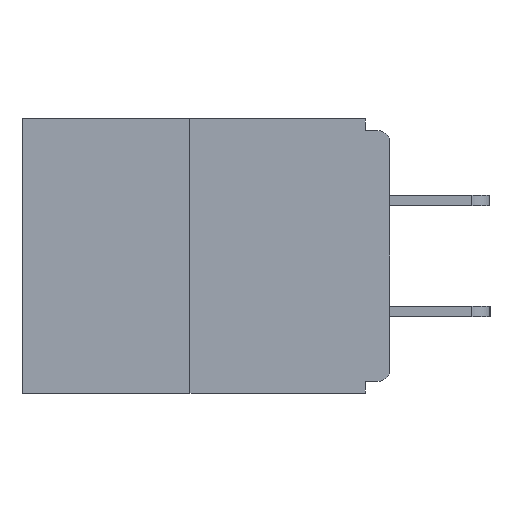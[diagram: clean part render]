
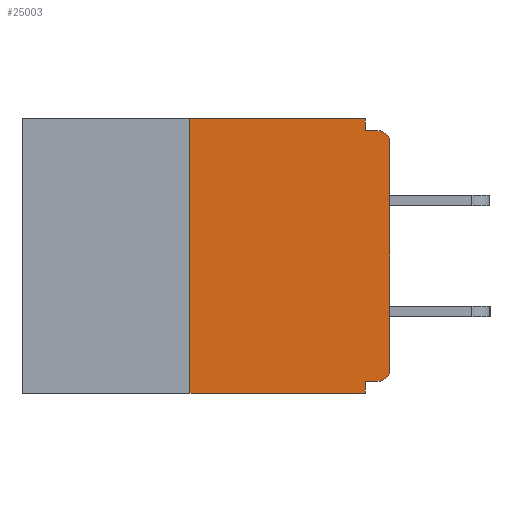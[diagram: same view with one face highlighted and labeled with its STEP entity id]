
A CAD part, left-side view. The second image highlights one B-rep face of the part: STEP entity #25003.
In plain terms, the highlighted planar face has unit normal (-1, 0, 0).
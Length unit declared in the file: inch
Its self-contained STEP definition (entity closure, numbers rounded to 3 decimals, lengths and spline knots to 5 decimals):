
#54 = VERTEX_POINT ( 'NONE', #17218 ) ;
#560 = VERTEX_POINT ( 'NONE', #18447 ) ;
#632 = CARTESIAN_POINT ( 'NONE',  ( 0., 0.25, -0.343 ) ) ;
#1004 = DIRECTION ( 'NONE',  ( 1., 0., 0. ) ) ;
#1020 = EDGE_CURVE ( 'NONE', #22884, #10326, #26032, .T. ) ;
#1209 = CARTESIAN_POINT ( 'NONE',  ( 0., 0.46, 0. ) ) ;
#1566 = ORIENTED_EDGE ( 'NONE', *, *, #19395, .F. ) ;
#1729 = CARTESIAN_POINT ( 'NONE',  ( 0., 0.015, -0.313 ) ) ;
#1945 = ORIENTED_EDGE ( 'NONE', *, *, #5148, .T. ) ;
#2674 = CARTESIAN_POINT ( 'NONE',  ( 0., 0., -0.328 ) ) ;
#2755 = DIRECTION ( 'NONE',  ( 0., 0., -1. ) ) ;
#2906 = LINE ( 'NONE', #23222, #14003 ) ;
#2956 = AXIS2_PLACEMENT_3D ( 'NONE', #24264, #5818, #22269 ) ;
#3060 = ORIENTED_EDGE ( 'NONE', *, *, #17266, .T. ) ;
#3271 = AXIS2_PLACEMENT_3D ( 'NONE', #5281, #1004, #7443 ) ;
#3299 = CARTESIAN_POINT ( 'NONE',  ( 0., 0., 0. ) ) ;
#3790 = VERTEX_POINT ( 'NONE', #10400 ) ;
#4500 = EDGE_CURVE ( 'NONE', #54, #8327, #11698, .T. ) ;
#4554 = VECTOR ( 'NONE', #18564, 39.37008 ) ;
#5148 = EDGE_CURVE ( 'NONE', #22478, #26376, #26455, .T. ) ;
#5281 = CARTESIAN_POINT ( 'NONE',  ( 0., 0.46, 0. ) ) ;
#5818 = DIRECTION ( 'NONE',  ( -1., 0., 0. ) ) ;
#7095 = VECTOR ( 'NONE', #7277, 39.37008 ) ;
#7277 = DIRECTION ( 'NONE',  ( 0., 0., -1. ) ) ;
#7323 = LINE ( 'NONE', #3299, #12209 ) ;
#7443 = DIRECTION ( 'NONE',  ( 0., 0., -1. ) ) ;
#7733 = EDGE_CURVE ( 'NONE', #8327, #25374, #17316, .T. ) ;
#7776 = CARTESIAN_POINT ( 'NONE',  ( 0., 0.46, -0.343 ) ) ;
#8327 = VERTEX_POINT ( 'NONE', #23055 ) ;
#8697 = EDGE_CURVE ( 'NONE', #22884, #560, #16909, .T. ) ;
#8846 = DIRECTION ( 'NONE',  ( 0., 1., 0. ) ) ;
#9107 = CARTESIAN_POINT ( 'NONE',  ( 0., 0., -0.015 ) ) ;
#9693 = ORIENTED_EDGE ( 'NONE', *, *, #1020, .T. ) ;
#10137 = VECTOR ( 'NONE', #20586, 39.37008 ) ;
#10212 = VECTOR ( 'NONE', #10858, 39.37008 ) ;
#10326 = VERTEX_POINT ( 'NONE', #21945 ) ;
#10337 = CARTESIAN_POINT ( 'NONE',  ( 0., 0.25, 0. ) ) ;
#10400 = CARTESIAN_POINT ( 'NONE',  ( 0., 0.25, 0. ) ) ;
#10466 = EDGE_CURVE ( 'NONE', #10326, #24249, #7323, .T. ) ;
#10858 = DIRECTION ( 'NONE',  ( 0., -1., 0. ) ) ;
#11034 = CARTESIAN_POINT ( 'NONE',  ( 0., 0., -0.03 ) ) ;
#11698 = LINE ( 'NONE', #23699, #7095 ) ;
#12086 = LINE ( 'NONE', #10337, #4554 ) ;
#12209 = VECTOR ( 'NONE', #12879, 39.37008 ) ;
#12280 = AXIS2_PLACEMENT_3D ( 'NONE', #1729, #13937, #18138 ) ;
#12622 = ORIENTED_EDGE ( 'NONE', *, *, #7733, .F. ) ;
#12879 = DIRECTION ( 'NONE',  ( 0., 0., 1. ) ) ;
#13374 = FACE_OUTER_BOUND ( 'NONE', #15676, .T. ) ;
#13558 = LINE ( 'NONE', #1209, #25602 ) ;
#13937 = DIRECTION ( 'NONE',  ( -1., 0., 0. ) ) ;
#14003 = VECTOR ( 'NONE', #2755, 39.37008 ) ;
#14537 = ORIENTED_EDGE ( 'NONE', *, *, #8697, .F. ) ;
#14550 = CIRCLE ( 'NONE', #2956, 0.015 ) ;
#15676 = EDGE_LOOP ( 'NONE', ( #16479, #1566, #1945, #21138, #14537, #9693, #23672, #3060, #12622, #23519 ) ) ;
#16479 = ORIENTED_EDGE ( 'NONE', *, *, #19364, .F. ) ;
#16909 = LINE ( 'NONE', #2674, #21766 ) ;
#17218 = CARTESIAN_POINT ( 'NONE',  ( 0., 0.031, 0. ) ) ;
#17266 = EDGE_CURVE ( 'NONE', #24249, #25374, #14550, .T. ) ;
#17316 = LINE ( 'NONE', #9107, #10212 ) ;
#17621 = DIRECTION ( 'NONE',  ( 0., -1., 0. ) ) ;
#17877 = CARTESIAN_POINT ( 'NONE',  ( 0., 0.015, -0.015 ) ) ;
#18138 = DIRECTION ( 'NONE',  ( 0., 0., -1. ) ) ;
#18189 = CARTESIAN_POINT ( 'NONE',  ( 0., 0.015, -0.328 ) ) ;
#18447 = CARTESIAN_POINT ( 'NONE',  ( 0., 0.031, -0.328 ) ) ;
#18564 = DIRECTION ( 'NONE',  ( 0., 0., 1. ) ) ;
#19364 = EDGE_CURVE ( 'NONE', #3790, #54, #13558, .T. ) ;
#19395 = EDGE_CURVE ( 'NONE', #22478, #3790, #12086, .T. ) ;
#19454 = PLANE ( 'NONE',  #3271 ) ;
#20586 = DIRECTION ( 'NONE',  ( 0., -1., 0. ) ) ;
#21138 = ORIENTED_EDGE ( 'NONE', *, *, #26142, .F. ) ;
#21766 = VECTOR ( 'NONE', #8846, 39.37008 ) ;
#21945 = CARTESIAN_POINT ( 'NONE',  ( 0., 0., -0.313 ) ) ;
#22269 = DIRECTION ( 'NONE',  ( 0., 0., -1. ) ) ;
#22478 = VERTEX_POINT ( 'NONE', #632 ) ;
#22884 = VERTEX_POINT ( 'NONE', #18189 ) ;
#23055 = CARTESIAN_POINT ( 'NONE',  ( 0., 0.031, -0.015 ) ) ;
#23222 = CARTESIAN_POINT ( 'NONE',  ( 0., 0.031, -0.343 ) ) ;
#23519 = ORIENTED_EDGE ( 'NONE', *, *, #4500, .F. ) ;
#23672 = ORIENTED_EDGE ( 'NONE', *, *, #10466, .T. ) ;
#23699 = CARTESIAN_POINT ( 'NONE',  ( 0., 0.031, 0. ) ) ;
#24249 = VERTEX_POINT ( 'NONE', #11034 ) ;
#24264 = CARTESIAN_POINT ( 'NONE',  ( 0., 0.015, -0.03 ) ) ;
#25003 = ADVANCED_FACE ( 'NONE', ( #13374 ), #19454, .F. ) ;
#25374 = VERTEX_POINT ( 'NONE', #17877 ) ;
#25602 = VECTOR ( 'NONE', #17621, 39.37008 ) ;
#25883 = CARTESIAN_POINT ( 'NONE',  ( 0., 0.031, -0.343 ) ) ;
#26032 = CIRCLE ( 'NONE', #12280, 0.015 ) ;
#26142 = EDGE_CURVE ( 'NONE', #560, #26376, #2906, .T. ) ;
#26376 = VERTEX_POINT ( 'NONE', #25883 ) ;
#26455 = LINE ( 'NONE', #7776, #10137 ) ;
